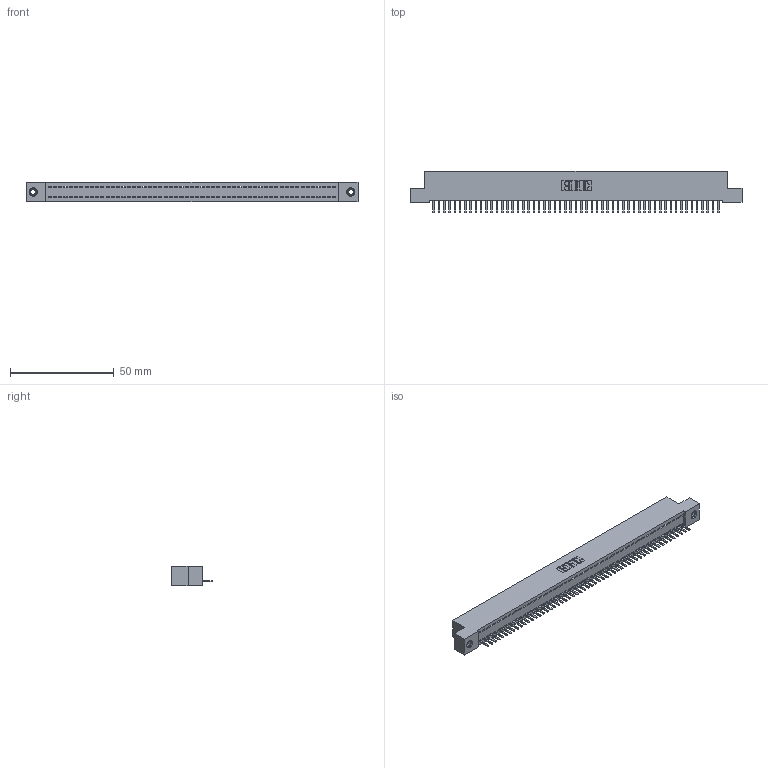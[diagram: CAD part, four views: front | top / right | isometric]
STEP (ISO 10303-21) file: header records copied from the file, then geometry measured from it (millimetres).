
FILE_DESCRIPTION (( 'STEP AP203' ), '1' );
FILE_NAME ('392-055-520-107.STEP', '2018-08-17T10:40:28', ( '' ), ( '' ), 'SwSTEP 2.0', 'SolidWorks 2016', '' );
FILE_SCHEMA (( 'CONFIG_CONTROL_DESIGN' ));
Length unit declared in the file: inch
Products named in the file (4): 392-055-520-107; 342 Part_TI; 345-292-001_345-293-120; 345-250-001_345-250-005-103
Assembly tree (58 placements, depth 2):
  392-055-520-107
    342 Part_TI
    345-292-001_345-293-120  x55
    345-250-001_345-250-005-103  x2
Bounding box: 160.02 x 20.02 x 9.4 mm (x, y, z)
Volume: 13907.5 mm3; surface area: 20191.5 mm2
Topology: 58 solids, 58 shells, 3580 faces, 10555 edges, 6882 vertices
Faces by surface type: plane 2518, cylinder 1046, cone 12, torus 4
Entity records: 33110 total; most frequent: CARTESIAN_POINT 5702, ORIENTED_EDGE 5674, DIRECTION 4805, EDGE_CURVE 2837, LINE 2685, VECTOR 2685, VERTEX_POINT 1884, AXIS2_PLACEMENT_3D 1060
